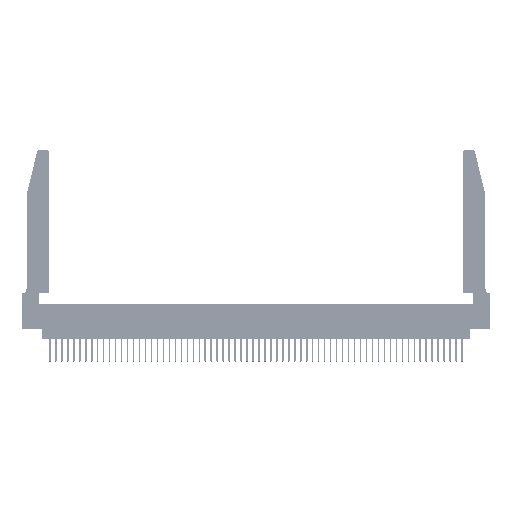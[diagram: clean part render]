
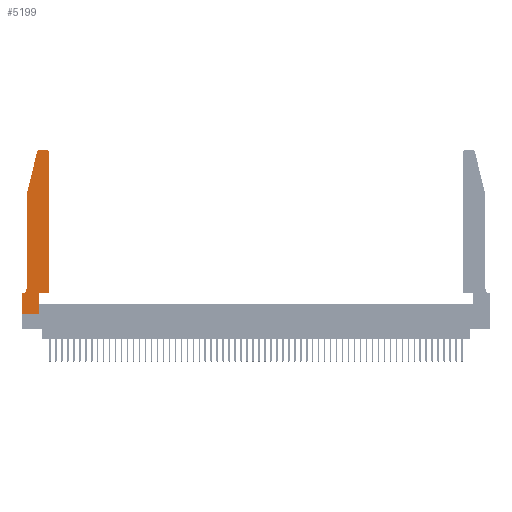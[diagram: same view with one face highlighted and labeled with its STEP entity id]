
A CAD part, top view. The second image highlights one B-rep face of the part: STEP entity #5199.
In plain terms, the highlighted planar face has unit normal (0, 0, 1).
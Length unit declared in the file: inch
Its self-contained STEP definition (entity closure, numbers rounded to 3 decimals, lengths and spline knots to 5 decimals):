
#11 = CARTESIAN_POINT ( 'NONE',  ( 0.0755, 2., 0.37 ) ) ;
#878 = VECTOR ( 'NONE', #49206, 39.37008 ) ;
#1710 = LINE ( 'NONE', #24682, #51876 ) ;
#2302 = CARTESIAN_POINT ( 'NONE',  ( 0., 0., 0.37 ) ) ;
#2577 = PLANE ( 'NONE',  #11799 ) ;
#2688 = FACE_OUTER_BOUND ( 'NONE', #35376, .T. ) ;
#3549 = LINE ( 'NONE', #14551, #878 ) ;
#4323 = AXIS2_PLACEMENT_3D ( 'NONE', #11482, #7328, #24764 ) ;
#4491 = VECTOR ( 'NONE', #42379, 39.37008 ) ;
#5199 = ADVANCED_FACE ( 'NONE', ( #2688 ), #2577, .T. ) ;
#5781 = CARTESIAN_POINT ( 'NONE',  ( 0.0755, 2., 0.37 ) ) ;
#6519 = ORIENTED_EDGE ( 'NONE', *, *, #16952, .T. ) ;
#6689 = CIRCLE ( 'NONE', #34745, 0.03 ) ;
#6835 = VECTOR ( 'NONE', #21102, 39.37008 ) ;
#7328 = DIRECTION ( 'NONE',  ( 0., 0., 1. ) ) ;
#8390 = ORIENTED_EDGE ( 'NONE', *, *, #22675, .T. ) ;
#8571 = CARTESIAN_POINT ( 'NONE',  ( 0.0755, 0.35, 0.37 ) ) ;
#9005 = CARTESIAN_POINT ( 'NONE',  ( 0.4205, 2.72, 0.37 ) ) ;
#9812 = CARTESIAN_POINT ( 'NONE',  ( 0.2865, 0.35, 0.37 ) ) ;
#9907 = LINE ( 'NONE', #44577, #55290 ) ;
#9963 = ORIENTED_EDGE ( 'NONE', *, *, #41429, .T. ) ;
#11482 = CARTESIAN_POINT ( 'NONE',  ( 0.284, 2.72, 0.37 ) ) ;
#11799 = AXIS2_PLACEMENT_3D ( 'NONE', #24750, #42166, #37266 ) ;
#12354 = CARTESIAN_POINT ( 'NONE',  ( 0.0055, 0.35, 0.37 ) ) ;
#14551 = CARTESIAN_POINT ( 'NONE',  ( 0.4505, 0.35, 0.37 ) ) ;
#14749 = VERTEX_POINT ( 'NONE', #15495 ) ;
#14895 = LINE ( 'NONE', #5781, #25085 ) ;
#15495 = CARTESIAN_POINT ( 'NONE',  ( 0., 0., 0.37 ) ) ;
#16952 = EDGE_CURVE ( 'NONE', #18820, #27725, #1710, .T. ) ;
#17894 = DIRECTION ( 'NONE',  ( 0., 0., 1. ) ) ;
#17900 = ORIENTED_EDGE ( 'NONE', *, *, #38823, .T. ) ;
#18684 = CIRCLE ( 'NONE', #4323, 0.03 ) ;
#18820 = VERTEX_POINT ( 'NONE', #37595 ) ;
#20611 = VERTEX_POINT ( 'NONE', #33477 ) ;
#20979 = EDGE_CURVE ( 'NONE', #39287, #42318, #6689, .T. ) ;
#21102 = DIRECTION ( 'NONE',  ( 0., -1., 0. ) ) ;
#21124 = CARTESIAN_POINT ( 'NONE',  ( 0.4505, 0.35, 0.37 ) ) ;
#22105 = CARTESIAN_POINT ( 'NONE',  ( 0.4205, 2.75, 0.37 ) ) ;
#22233 = DIRECTION ( 'NONE',  ( 1., 0., 0. ) ) ;
#22675 = EDGE_CURVE ( 'NONE', #27725, #29843, #24126, .T. ) ;
#22957 = DIRECTION ( 'NONE',  ( -1., 0., 0. ) ) ;
#23290 = CARTESIAN_POINT ( 'NONE',  ( 0.284, 2.75, 0.37 ) ) ;
#24126 = LINE ( 'NONE', #21124, #4491 ) ;
#24229 = VECTOR ( 'NONE', #46535, 39.37008 ) ;
#24682 = CARTESIAN_POINT ( 'NONE',  ( 0.2865, 0.35, 0.37 ) ) ;
#24750 = CARTESIAN_POINT ( 'NONE',  ( 0., 0.35, 0.37 ) ) ;
#24764 = DIRECTION ( 'NONE',  ( 1., 0., 0. ) ) ;
#25085 = VECTOR ( 'NONE', #40831, 39.37008 ) ;
#25867 = ORIENTED_EDGE ( 'NONE', *, *, #26924, .T. ) ;
#26092 = EDGE_CURVE ( 'NONE', #54353, #55170, #18684, .T. ) ;
#26924 = EDGE_CURVE ( 'NONE', #51611, #30119, #43059, .T. ) ;
#27185 = LINE ( 'NONE', #42723, #6835 ) ;
#27703 = VERTEX_POINT ( 'NONE', #11 ) ;
#27725 = VERTEX_POINT ( 'NONE', #9812 ) ;
#27766 = LINE ( 'NONE', #2302, #34538 ) ;
#27768 = ORIENTED_EDGE ( 'NONE', *, *, #20979, .T. ) ;
#29540 = DIRECTION ( 'NONE',  ( 0., 0., -1. ) ) ;
#29843 = VERTEX_POINT ( 'NONE', #54186 ) ;
#30000 = AXIS2_PLACEMENT_3D ( 'NONE', #50583, #29540, #38297 ) ;
#30119 = VERTEX_POINT ( 'NONE', #55871 ) ;
#31765 = CARTESIAN_POINT ( 'NONE',  ( 0.25487, 2.72718, 0.37 ) ) ;
#32643 = EDGE_CURVE ( 'NONE', #20611, #51611, #49085, .T. ) ;
#33004 = DIRECTION ( 'NONE',  ( 1., 0., 0. ) ) ;
#33477 = CARTESIAN_POINT ( 'NONE',  ( 0.0755, 0.42, 0.37 ) ) ;
#34173 = CARTESIAN_POINT ( 'NONE',  ( 0.4505, 2.72, 0.37 ) ) ;
#34538 = VECTOR ( 'NONE', #33004, 39.37008 ) ;
#34745 = AXIS2_PLACEMENT_3D ( 'NONE', #9005, #17894, #22233 ) ;
#35376 = EDGE_LOOP ( 'NONE', ( #9963, #39052, #38948, #17900, #38452, #25867, #45623, #46611, #6519, #8390, #44418, #27768 ) ) ;
#37266 = DIRECTION ( 'NONE',  ( 1., 0., 0. ) ) ;
#37595 = CARTESIAN_POINT ( 'NONE',  ( 0.2865, 0., 0.37 ) ) ;
#37654 = CARTESIAN_POINT ( 'NONE',  ( 0.0755, 2., 0.37 ) ) ;
#38131 = EDGE_CURVE ( 'NONE', #30119, #14749, #27185, .T. ) ;
#38297 = DIRECTION ( 'NONE',  ( -1., 0., 0. ) ) ;
#38452 = ORIENTED_EDGE ( 'NONE', *, *, #32643, .T. ) ;
#38823 = EDGE_CURVE ( 'NONE', #27703, #20611, #14895, .T. ) ;
#38922 = DIRECTION ( 'NONE',  ( -1., 0., 0. ) ) ;
#38948 = ORIENTED_EDGE ( 'NONE', *, *, #52901, .T. ) ;
#39052 = ORIENTED_EDGE ( 'NONE', *, *, #26092, .T. ) ;
#39287 = VERTEX_POINT ( 'NONE', #34173 ) ;
#39495 = EDGE_CURVE ( 'NONE', #14749, #18820, #27766, .T. ) ;
#40831 = DIRECTION ( 'NONE',  ( 0., -1., 0. ) ) ;
#41429 = EDGE_CURVE ( 'NONE', #42318, #54353, #9907, .T. ) ;
#42094 = DIRECTION ( 'NONE',  ( 0., 1., 0. ) ) ;
#42166 = DIRECTION ( 'NONE',  ( 0., 0., 1. ) ) ;
#42318 = VERTEX_POINT ( 'NONE', #22105 ) ;
#42379 = DIRECTION ( 'NONE',  ( 1., 0., 0. ) ) ;
#42723 = CARTESIAN_POINT ( 'NONE',  ( 0., 0., 0.37 ) ) ;
#43059 = LINE ( 'NONE', #8571, #52516 ) ;
#44418 = ORIENTED_EDGE ( 'NONE', *, *, #49146, .T. ) ;
#44577 = CARTESIAN_POINT ( 'NONE',  ( 0.2605, 2.75, 0.37 ) ) ;
#45623 = ORIENTED_EDGE ( 'NONE', *, *, #38131, .T. ) ;
#46535 = DIRECTION ( 'NONE',  ( -0.239, -0.971, 0. ) ) ;
#46611 = ORIENTED_EDGE ( 'NONE', *, *, #39495, .T. ) ;
#49085 = CIRCLE ( 'NONE', #30000, 0.07 ) ;
#49146 = EDGE_CURVE ( 'NONE', #29843, #39287, #3549, .T. ) ;
#49206 = DIRECTION ( 'NONE',  ( 0., 1., 0. ) ) ;
#50583 = CARTESIAN_POINT ( 'NONE',  ( 0.0055, 0.42, 0.37 ) ) ;
#51611 = VERTEX_POINT ( 'NONE', #12354 ) ;
#51876 = VECTOR ( 'NONE', #42094, 39.37008 ) ;
#52021 = LINE ( 'NONE', #37654, #24229 ) ;
#52516 = VECTOR ( 'NONE', #38922, 39.37008 ) ;
#52901 = EDGE_CURVE ( 'NONE', #55170, #27703, #52021, .T. ) ;
#54186 = CARTESIAN_POINT ( 'NONE',  ( 0.4505, 0.35, 0.37 ) ) ;
#54353 = VERTEX_POINT ( 'NONE', #23290 ) ;
#55170 = VERTEX_POINT ( 'NONE', #31765 ) ;
#55290 = VECTOR ( 'NONE', #22957, 39.37008 ) ;
#55871 = CARTESIAN_POINT ( 'NONE',  ( 0., 0.35, 0.37 ) ) ;
